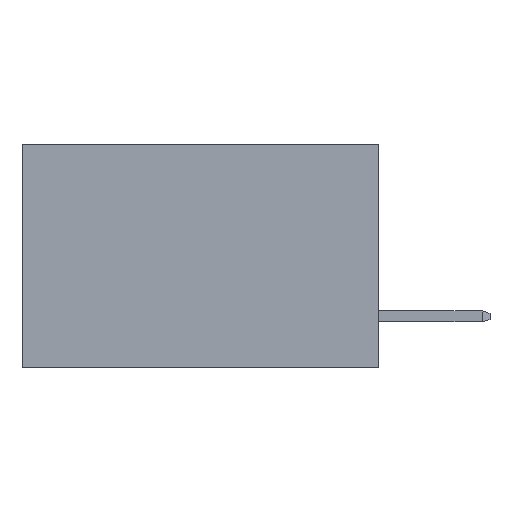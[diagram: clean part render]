
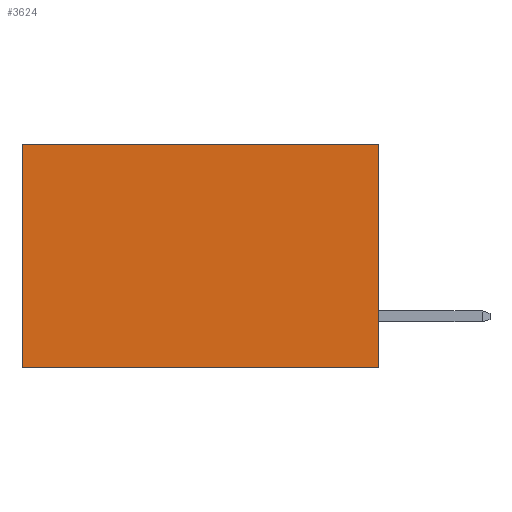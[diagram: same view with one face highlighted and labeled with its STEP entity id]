
A CAD part, left-side view. The second image highlights one B-rep face of the part: STEP entity #3624.
In plain terms, the highlighted planar face has unit normal (-1, 0, 0).
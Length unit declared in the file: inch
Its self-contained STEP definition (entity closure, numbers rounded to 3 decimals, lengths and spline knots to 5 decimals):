
#49 = ORIENTED_EDGE ( 'NONE', *, *, #8986, .T. ) ;
#197 = VECTOR ( 'NONE', #4576, 39.37008 ) ;
#693 = EDGE_CURVE ( 'NONE', #5861, #5674, #6765, .T. ) ;
#900 = EDGE_CURVE ( 'NONE', #5861, #7721, #7372, .T. ) ;
#1117 = DIRECTION ( 'NONE',  ( 0., 1., 0. ) ) ;
#1446 = EDGE_LOOP ( 'NONE', ( #49, #4645, #7224, #7911 ) ) ;
#2398 = VECTOR ( 'NONE', #9750, 39.37008 ) ;
#2469 = LINE ( 'NONE', #4804, #197 ) ;
#2659 = CARTESIAN_POINT ( 'NONE',  ( 0.277, 0., -0.37 ) ) ;
#3624 = ADVANCED_FACE ( 'NONE', ( #5630 ), #6995, .F. ) ;
#4523 = LINE ( 'NONE', #5872, #2398 ) ;
#4576 = DIRECTION ( 'NONE',  ( 0., 1., 0. ) ) ;
#4645 = ORIENTED_EDGE ( 'NONE', *, *, #5419, .F. ) ;
#4691 = VECTOR ( 'NONE', #5607, 39.37008 ) ;
#4804 = CARTESIAN_POINT ( 'NONE',  ( 0.277, 0., -0.37 ) ) ;
#5053 = VECTOR ( 'NONE', #1117, 39.37008 ) ;
#5419 = EDGE_CURVE ( 'NONE', #5674, #9362, #2469, .T. ) ;
#5607 = DIRECTION ( 'NONE',  ( 0., 0., -1. ) ) ;
#5630 = FACE_OUTER_BOUND ( 'NONE', #1446, .T. ) ;
#5674 = VERTEX_POINT ( 'NONE', #9011 ) ;
#5861 = VERTEX_POINT ( 'NONE', #9520 ) ;
#5872 = CARTESIAN_POINT ( 'NONE',  ( 0.277, 0.59, -0.37 ) ) ;
#6572 = CARTESIAN_POINT ( 'NONE',  ( 0.277, 0.59, 0. ) ) ;
#6765 = LINE ( 'NONE', #2659, #4691 ) ;
#6940 = DIRECTION ( 'NONE',  ( 0., 0., -1. ) ) ;
#6949 = DIRECTION ( 'NONE',  ( 1., 0., 0. ) ) ;
#6971 = CARTESIAN_POINT ( 'NONE',  ( 0.277, 0., -0.37 ) ) ;
#6995 = PLANE ( 'NONE',  #7908 ) ;
#7224 = ORIENTED_EDGE ( 'NONE', *, *, #693, .F. ) ;
#7372 = LINE ( 'NONE', #7646, #5053 ) ;
#7646 = CARTESIAN_POINT ( 'NONE',  ( 0.277, 0., 0. ) ) ;
#7721 = VERTEX_POINT ( 'NONE', #6572 ) ;
#7908 = AXIS2_PLACEMENT_3D ( 'NONE', #6971, #6949, #6940 ) ;
#7911 = ORIENTED_EDGE ( 'NONE', *, *, #900, .T. ) ;
#8986 = EDGE_CURVE ( 'NONE', #7721, #9362, #4523, .T. ) ;
#9011 = CARTESIAN_POINT ( 'NONE',  ( 0.277, 0., -0.37 ) ) ;
#9362 = VERTEX_POINT ( 'NONE', #10335 ) ;
#9520 = CARTESIAN_POINT ( 'NONE',  ( 0.277, 0., 0. ) ) ;
#9750 = DIRECTION ( 'NONE',  ( 0., 0., -1. ) ) ;
#10335 = CARTESIAN_POINT ( 'NONE',  ( 0.277, 0.59, -0.37 ) ) ;
